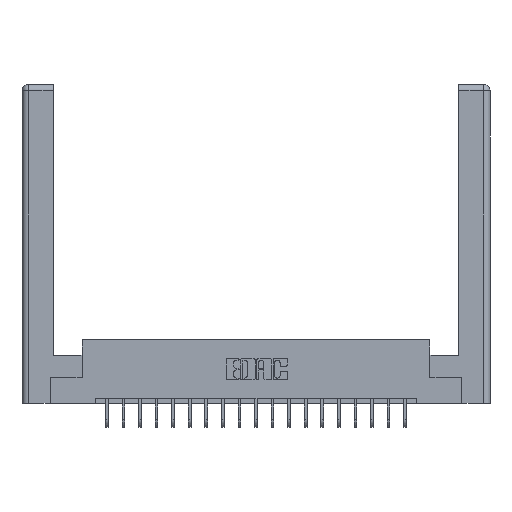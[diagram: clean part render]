
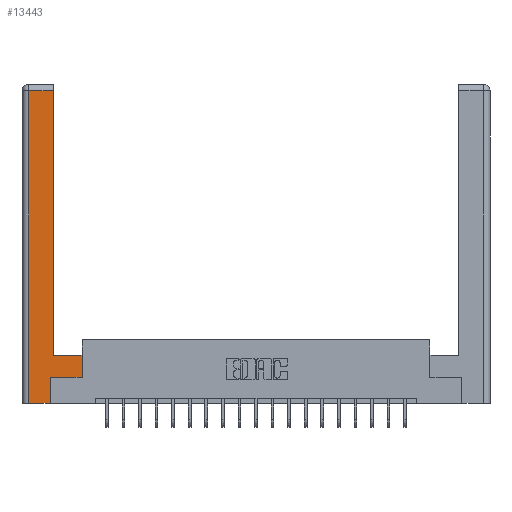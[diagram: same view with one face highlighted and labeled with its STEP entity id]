
A CAD part, top view. The second image highlights one B-rep face of the part: STEP entity #13443.
In plain terms, the highlighted planar face has unit normal (0, 0, 1).
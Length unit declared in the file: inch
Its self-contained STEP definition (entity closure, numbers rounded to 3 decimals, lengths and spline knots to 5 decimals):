
#427 = CARTESIAN_POINT ( 'NONE',  ( 0.295, 2.94, 0. ) ) ;
#797 = VECTOR ( 'NONE', #16139, 39.37008 ) ;
#1158 = LINE ( 'NONE', #1806, #3563 ) ;
#1332 = CARTESIAN_POINT ( 'NONE',  ( 0., 0., 0. ) ) ;
#1792 = EDGE_CURVE ( 'NONE', #2584, #21152, #1882, .T. ) ;
#1806 = CARTESIAN_POINT ( 'NONE',  ( 0.265, 0.245, 0. ) ) ;
#1882 = LINE ( 'NONE', #5470, #18465 ) ;
#2120 = CARTESIAN_POINT ( 'NONE',  ( 0.265, 0., 0. ) ) ;
#2305 = CARTESIAN_POINT ( 'NONE',  ( 0.565, 0.45, 0. ) ) ;
#2344 = VERTEX_POINT ( 'NONE', #18628 ) ;
#2584 = VERTEX_POINT ( 'NONE', #2305 ) ;
#3322 = CARTESIAN_POINT ( 'NONE',  ( 0.565, 0.245, 0. ) ) ;
#3563 = VECTOR ( 'NONE', #19011, 39.37008 ) ;
#3605 = CARTESIAN_POINT ( 'NONE',  ( 0.565, 0.45, 0. ) ) ;
#4404 = VECTOR ( 'NONE', #8460, 39.37008 ) ;
#5063 = VERTEX_POINT ( 'NONE', #13512 ) ;
#5470 = CARTESIAN_POINT ( 'NONE',  ( 0.295, 0.45, 0. ) ) ;
#5513 = VECTOR ( 'NONE', #8117, 39.37008 ) ;
#5551 = EDGE_CURVE ( 'NONE', #13188, #2584, #8935, .T. ) ;
#5556 = VECTOR ( 'NONE', #15170, 39.37008 ) ;
#5747 = ORIENTED_EDGE ( 'NONE', *, *, #19578, .T. ) ;
#6784 = VECTOR ( 'NONE', #7034, 39.37008 ) ;
#7034 = DIRECTION ( 'NONE',  ( 0., 1., 0. ) ) ;
#7078 = VERTEX_POINT ( 'NONE', #427 ) ;
#7339 = CARTESIAN_POINT ( 'NONE',  ( 0.0615, 2.94, 0. ) ) ;
#7619 = EDGE_CURVE ( 'NONE', #2344, #15502, #21242, .T. ) ;
#8117 = DIRECTION ( 'NONE',  ( 0., 1., 0. ) ) ;
#8226 = EDGE_CURVE ( 'NONE', #21725, #2344, #8921, .T. ) ;
#8284 = EDGE_LOOP ( 'NONE', ( #19349, #5747, #14546, #16912, #20966, #21753, #17739, #8688 ) ) ;
#8347 = EDGE_CURVE ( 'NONE', #15502, #5063, #1158, .T. ) ;
#8460 = DIRECTION ( 'NONE',  ( 0., -1., 0. ) ) ;
#8688 = ORIENTED_EDGE ( 'NONE', *, *, #1792, .T. ) ;
#8828 = DIRECTION ( 'NONE',  ( 1., 0., 0. ) ) ;
#8921 = LINE ( 'NONE', #13718, #4404 ) ;
#8935 = LINE ( 'NONE', #3605, #6784 ) ;
#9577 = DIRECTION ( 'NONE',  ( -1., 0., 0. ) ) ;
#9850 = PLANE ( 'NONE',  #12576 ) ;
#11654 = LINE ( 'NONE', #17998, #5513 ) ;
#12305 = CARTESIAN_POINT ( 'NONE',  ( 0.295, 0.45, 0. ) ) ;
#12576 = AXIS2_PLACEMENT_3D ( 'NONE', #1332, #13313, #9577 ) ;
#13188 = VERTEX_POINT ( 'NONE', #20401 ) ;
#13313 = DIRECTION ( 'NONE',  ( 0., 0., -1. ) ) ;
#13443 = ADVANCED_FACE ( 'NONE', ( #17617 ), #9850, .F. ) ;
#13512 = CARTESIAN_POINT ( 'NONE',  ( 0.265, 0.245, 0. ) ) ;
#13718 = CARTESIAN_POINT ( 'NONE',  ( 0.0615, 0., 0. ) ) ;
#13995 = EDGE_CURVE ( 'NONE', #5063, #13188, #15470, .T. ) ;
#14458 = CARTESIAN_POINT ( 'NONE',  ( 0.0615, 2.94, 0. ) ) ;
#14546 = ORIENTED_EDGE ( 'NONE', *, *, #8226, .T. ) ;
#14548 = EDGE_CURVE ( 'NONE', #21152, #7078, #11654, .T. ) ;
#14808 = CARTESIAN_POINT ( 'NONE',  ( 0.265, 0., 0. ) ) ;
#15170 = DIRECTION ( 'NONE',  ( 1., 0., 0. ) ) ;
#15470 = LINE ( 'NONE', #3322, #5556 ) ;
#15502 = VERTEX_POINT ( 'NONE', #14808 ) ;
#16139 = DIRECTION ( 'NONE',  ( -1., 0., 0. ) ) ;
#16912 = ORIENTED_EDGE ( 'NONE', *, *, #7619, .T. ) ;
#17617 = FACE_OUTER_BOUND ( 'NONE', #8284, .T. ) ;
#17739 = ORIENTED_EDGE ( 'NONE', *, *, #5551, .T. ) ;
#17998 = CARTESIAN_POINT ( 'NONE',  ( 0.295, 3., 0. ) ) ;
#18465 = VECTOR ( 'NONE', #20554, 39.37008 ) ;
#18628 = CARTESIAN_POINT ( 'NONE',  ( 0.0615, 0., 0. ) ) ;
#19011 = DIRECTION ( 'NONE',  ( 0., 1., 0. ) ) ;
#19349 = ORIENTED_EDGE ( 'NONE', *, *, #14548, .T. ) ;
#19578 = EDGE_CURVE ( 'NONE', #7078, #21725, #21881, .T. ) ;
#20401 = CARTESIAN_POINT ( 'NONE',  ( 0.565, 0.245, 0. ) ) ;
#20554 = DIRECTION ( 'NONE',  ( -1., 0., 0. ) ) ;
#20966 = ORIENTED_EDGE ( 'NONE', *, *, #8347, .T. ) ;
#21152 = VERTEX_POINT ( 'NONE', #12305 ) ;
#21242 = LINE ( 'NONE', #2120, #21521 ) ;
#21521 = VECTOR ( 'NONE', #8828, 39.37008 ) ;
#21725 = VERTEX_POINT ( 'NONE', #7339 ) ;
#21753 = ORIENTED_EDGE ( 'NONE', *, *, #13995, .T. ) ;
#21881 = LINE ( 'NONE', #14458, #797 ) ;
